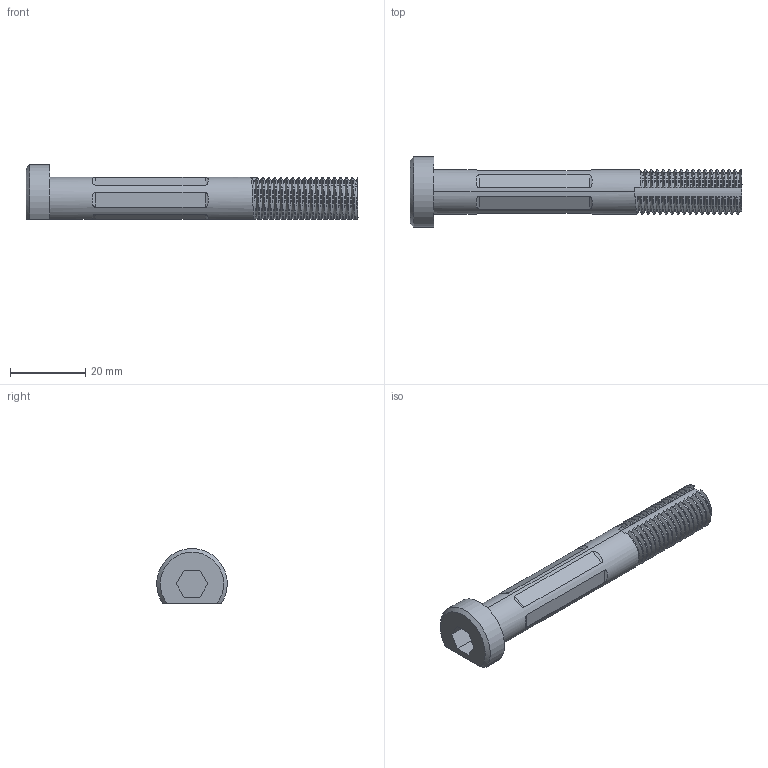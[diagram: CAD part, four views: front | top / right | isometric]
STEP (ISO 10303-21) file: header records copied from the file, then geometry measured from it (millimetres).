
FILE_DESCRIPTION (( 'STEP AP203' ), '1' );
FILE_NAME ('AF-HF-LR-PRT-006-STEP.STEP', '2020-10-30T14:19:18', ( '' ), ( '' ), 'SwSTEP 2.0', 'SolidWorks 2018', '' );
FILE_SCHEMA (( 'CONFIG_CONTROL_DESIGN' ));
Products named in the file (1): AF-HF-LR-PRT-006-STEP
Bounding box: 88.24 x 18.69 x 14.53 mm (x, y, z)
Volume: 9263.5 mm3; surface area: 4518.9 mm2
Topology: 1 solids, 1 shells, 166 faces, 461 edges, 302 vertices
Faces by surface type: plane 61, bspline 54, cylinder 50, cone 1
Entity records: 37292 total; most frequent: CARTESIAN_POINT 33921, ORIENTED_EDGE 922, EDGE_CURVE 461, DIRECTION 430, VERTEX_POINT 302, LINE 184, VECTOR 184, EDGE_LOOP 171
